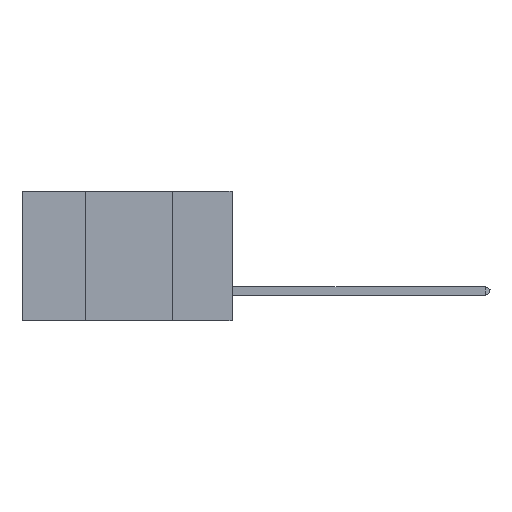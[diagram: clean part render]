
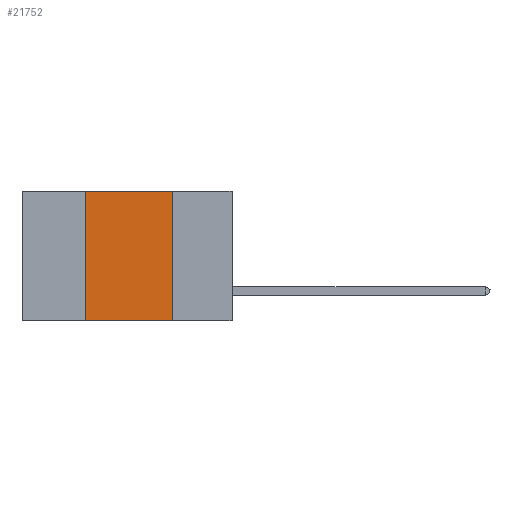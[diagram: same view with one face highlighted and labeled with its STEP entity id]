
A CAD part, left-side view. The second image highlights one B-rep face of the part: STEP entity #21752.
In plain terms, the highlighted planar face has unit normal (-1, 0, 0).
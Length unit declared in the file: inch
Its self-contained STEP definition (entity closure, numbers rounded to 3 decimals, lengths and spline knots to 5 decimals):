
#1195 = EDGE_CURVE ( 'NONE', #2514, #8849, #4438, .T. ) ;
#2514 = VERTEX_POINT ( 'NONE', #4827 ) ;
#3237 = ORIENTED_EDGE ( 'NONE', *, *, #1195, .F. ) ;
#3876 = DIRECTION ( 'NONE',  ( 0., -1., 0. ) ) ;
#4105 = VECTOR ( 'NONE', #27802, 39.37008 ) ;
#4438 = LINE ( 'NONE', #24070, #25827 ) ;
#4827 = CARTESIAN_POINT ( 'NONE',  ( 0., 0.42, 0. ) ) ;
#5533 = EDGE_CURVE ( 'NONE', #19403, #2514, #16865, .T. ) ;
#7010 = EDGE_CURVE ( 'NONE', #19403, #8441, #16424, .T. ) ;
#7042 = CARTESIAN_POINT ( 'NONE',  ( 0., 0.17, 0. ) ) ;
#8280 = VECTOR ( 'NONE', #24686, 39.37008 ) ;
#8441 = VERTEX_POINT ( 'NONE', #13218 ) ;
#8849 = VERTEX_POINT ( 'NONE', #7042 ) ;
#10907 = VECTOR ( 'NONE', #27134, 39.37008 ) ;
#11149 = AXIS2_PLACEMENT_3D ( 'NONE', #18630, #11887, #20854 ) ;
#11713 = ORIENTED_EDGE ( 'NONE', *, *, #27459, .F. ) ;
#11887 = DIRECTION ( 'NONE',  ( 1., 0., 0. ) ) ;
#13218 = CARTESIAN_POINT ( 'NONE',  ( 0., 0.17, -0.37 ) ) ;
#14048 = PLANE ( 'NONE',  #11149 ) ;
#14287 = LINE ( 'NONE', #20260, #8280 ) ;
#16020 = EDGE_LOOP ( 'NONE', ( #11713, #3237, #26688, #18446 ) ) ;
#16424 = LINE ( 'NONE', #23215, #4105 ) ;
#16865 = LINE ( 'NONE', #20169, #10907 ) ;
#18446 = ORIENTED_EDGE ( 'NONE', *, *, #7010, .T. ) ;
#18630 = CARTESIAN_POINT ( 'NONE',  ( 0., 0.6, 0. ) ) ;
#18703 = CARTESIAN_POINT ( 'NONE',  ( 0., 0.42, -0.37 ) ) ;
#19403 = VERTEX_POINT ( 'NONE', #18703 ) ;
#20169 = CARTESIAN_POINT ( 'NONE',  ( 0., 0.42, 0. ) ) ;
#20260 = CARTESIAN_POINT ( 'NONE',  ( 0., 0.17, 0. ) ) ;
#20854 = DIRECTION ( 'NONE',  ( 0., 0., -1. ) ) ;
#21752 = ADVANCED_FACE ( 'NONE', ( #23980 ), #14048, .F. ) ;
#23215 = CARTESIAN_POINT ( 'NONE',  ( 0., 0.6, -0.37 ) ) ;
#23980 = FACE_OUTER_BOUND ( 'NONE', #16020, .T. ) ;
#24070 = CARTESIAN_POINT ( 'NONE',  ( 0., 0.6, 0. ) ) ;
#24686 = DIRECTION ( 'NONE',  ( 0., 0., -1. ) ) ;
#25827 = VECTOR ( 'NONE', #3876, 39.37008 ) ;
#26688 = ORIENTED_EDGE ( 'NONE', *, *, #5533, .F. ) ;
#27134 = DIRECTION ( 'NONE',  ( 0., 0., 1. ) ) ;
#27459 = EDGE_CURVE ( 'NONE', #8849, #8441, #14287, .T. ) ;
#27802 = DIRECTION ( 'NONE',  ( 0., -1., 0. ) ) ;
